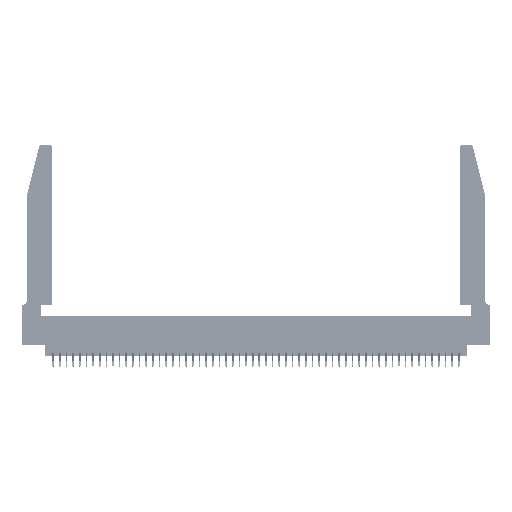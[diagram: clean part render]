
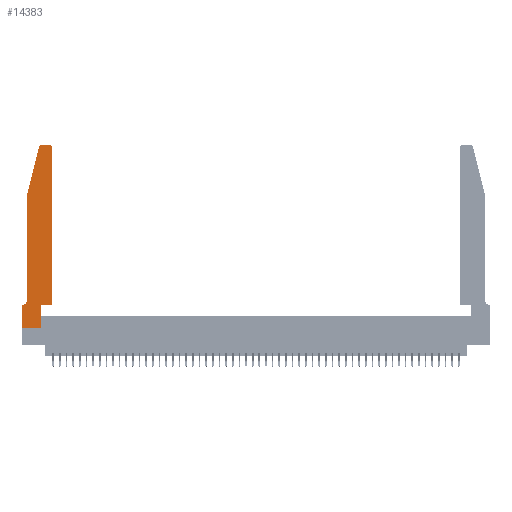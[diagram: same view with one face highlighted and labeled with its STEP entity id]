
A CAD part, top view. The second image highlights one B-rep face of the part: STEP entity #14383.
In plain terms, the highlighted planar face has unit normal (0, 0, 1).
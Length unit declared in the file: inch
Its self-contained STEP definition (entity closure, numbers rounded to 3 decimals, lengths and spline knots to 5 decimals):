
#1143 = CARTESIAN_POINT ( 'NONE',  ( 0.0755, 0.42, 0.37 ) ) ;
#2028 = DIRECTION ( 'NONE',  ( 0., 0., 1. ) ) ;
#2454 = ORIENTED_EDGE ( 'NONE', *, *, #25500, .T. ) ;
#2804 = EDGE_CURVE ( 'NONE', #31551, #34069, #6048, .T. ) ;
#2999 = EDGE_CURVE ( 'NONE', #5191, #14008, #40572, .T. ) ;
#3067 = DIRECTION ( 'NONE',  ( -0.239, -0.971, 0. ) ) ;
#3151 = CARTESIAN_POINT ( 'NONE',  ( 0.0755, 0.35, 0.37 ) ) ;
#3518 = AXIS2_PLACEMENT_3D ( 'NONE', #34191, #10553, #38124 ) ;
#3556 = VERTEX_POINT ( 'NONE', #25997 ) ;
#3999 = EDGE_LOOP ( 'NONE', ( #34614, #4310, #8051, #2454, #29791, #9944, #42616, #12453, #47513, #5003, #26138, #18088 ) ) ;
#4310 = ORIENTED_EDGE ( 'NONE', *, *, #16962, .T. ) ;
#4603 = AXIS2_PLACEMENT_3D ( 'NONE', #25837, #2028, #29796 ) ;
#5003 = ORIENTED_EDGE ( 'NONE', *, *, #2804, .T. ) ;
#5191 = VERTEX_POINT ( 'NONE', #32025 ) ;
#6048 = LINE ( 'NONE', #21754, #7297 ) ;
#6555 = PLANE ( 'NONE',  #3518 ) ;
#6983 = CARTESIAN_POINT ( 'NONE',  ( 0.2605, 2.75, 0.37 ) ) ;
#7101 = EDGE_CURVE ( 'NONE', #43563, #31551, #26178, .T. ) ;
#7297 = VECTOR ( 'NONE', #9914, 39.37008 ) ;
#7477 = LINE ( 'NONE', #26869, #37720 ) ;
#8051 = ORIENTED_EDGE ( 'NONE', *, *, #47389, .T. ) ;
#8503 = DIRECTION ( 'NONE',  ( 0., 0., -1. ) ) ;
#8507 = VERTEX_POINT ( 'NONE', #35699 ) ;
#9914 = DIRECTION ( 'NONE',  ( 1., 0., 0. ) ) ;
#9944 = ORIENTED_EDGE ( 'NONE', *, *, #44230, .T. ) ;
#10089 = EDGE_CURVE ( 'NONE', #35684, #3556, #35107, .T. ) ;
#10257 = CARTESIAN_POINT ( 'NONE',  ( 0.4205, 2.72, 0.37 ) ) ;
#10553 = DIRECTION ( 'NONE',  ( 0., 0., 1. ) ) ;
#10909 = CARTESIAN_POINT ( 'NONE',  ( 0.0755, 2., 0.37 ) ) ;
#11151 = DIRECTION ( 'NONE',  ( 0., 1., 0. ) ) ;
#12453 = ORIENTED_EDGE ( 'NONE', *, *, #48318, .T. ) ;
#12733 = LINE ( 'NONE', #19677, #32492 ) ;
#14008 = VERTEX_POINT ( 'NONE', #43639 ) ;
#14261 = DIRECTION ( 'NONE',  ( 1., 0., 0. ) ) ;
#14383 = ADVANCED_FACE ( 'NONE', ( #47519 ), #6555, .T. ) ;
#15183 = DIRECTION ( 'NONE',  ( -1., 0., 0. ) ) ;
#16836 = VERTEX_POINT ( 'NONE', #1143 ) ;
#16962 = EDGE_CURVE ( 'NONE', #3556, #35277, #45431, .T. ) ;
#18088 = ORIENTED_EDGE ( 'NONE', *, *, #19020, .T. ) ;
#18492 = VECTOR ( 'NONE', #22938, 39.37008 ) ;
#18789 = CARTESIAN_POINT ( 'NONE',  ( 0.4205, 2.75, 0.37 ) ) ;
#18971 = CARTESIAN_POINT ( 'NONE',  ( 0.25487, 2.72718, 0.37 ) ) ;
#18990 = CARTESIAN_POINT ( 'NONE',  ( 0.2865, 0.35, 0.37 ) ) ;
#19020 = EDGE_CURVE ( 'NONE', #8507, #35684, #40999, .T. ) ;
#19677 = CARTESIAN_POINT ( 'NONE',  ( 0.4505, 0.35, 0.37 ) ) ;
#21297 = EDGE_CURVE ( 'NONE', #16836, #31714, #43798, .T. ) ;
#21754 = CARTESIAN_POINT ( 'NONE',  ( 0.4505, 0.35, 0.37 ) ) ;
#22223 = DIRECTION ( 'NONE',  ( 0., -1., 0. ) ) ;
#22422 = DIRECTION ( 'NONE',  ( 1., 0., 0. ) ) ;
#22938 = DIRECTION ( 'NONE',  ( 0., -1., 0. ) ) ;
#25500 = EDGE_CURVE ( 'NONE', #47380, #16836, #27535, .T. ) ;
#25837 = CARTESIAN_POINT ( 'NONE',  ( 0.284, 2.72, 0.37 ) ) ;
#25993 = AXIS2_PLACEMENT_3D ( 'NONE', #10257, #37832, #14261 ) ;
#25997 = CARTESIAN_POINT ( 'NONE',  ( 0.284, 2.75, 0.37 ) ) ;
#26138 = ORIENTED_EDGE ( 'NONE', *, *, #37621, .T. ) ;
#26178 = LINE ( 'NONE', #18990, #36567 ) ;
#26296 = VECTOR ( 'NONE', #22223, 39.37008 ) ;
#26869 = CARTESIAN_POINT ( 'NONE',  ( 0.0755, 2., 0.37 ) ) ;
#27245 = VECTOR ( 'NONE', #22422, 39.37008 ) ;
#27535 = LINE ( 'NONE', #29981, #26296 ) ;
#29791 = ORIENTED_EDGE ( 'NONE', *, *, #21297, .T. ) ;
#29796 = DIRECTION ( 'NONE',  ( 1., 0., 0. ) ) ;
#29981 = CARTESIAN_POINT ( 'NONE',  ( 0.0755, 2., 0.37 ) ) ;
#31551 = VERTEX_POINT ( 'NONE', #49388 ) ;
#31714 = VERTEX_POINT ( 'NONE', #38798 ) ;
#32025 = CARTESIAN_POINT ( 'NONE',  ( 0., 0.35, 0.37 ) ) ;
#32199 = CARTESIAN_POINT ( 'NONE',  ( 0.0055, 0.42, 0.37 ) ) ;
#32492 = VECTOR ( 'NONE', #50989, 39.37008 ) ;
#33883 = VECTOR ( 'NONE', #38519, 39.37008 ) ;
#34069 = VERTEX_POINT ( 'NONE', #44837 ) ;
#34191 = CARTESIAN_POINT ( 'NONE',  ( 0., 0.35, 0.37 ) ) ;
#34231 = CARTESIAN_POINT ( 'NONE',  ( 0., 0., 0.37 ) ) ;
#34614 = ORIENTED_EDGE ( 'NONE', *, *, #10089, .T. ) ;
#35107 = LINE ( 'NONE', #6983, #33883 ) ;
#35277 = VERTEX_POINT ( 'NONE', #18971 ) ;
#35684 = VERTEX_POINT ( 'NONE', #18789 ) ;
#35699 = CARTESIAN_POINT ( 'NONE',  ( 0.4505, 2.72, 0.37 ) ) ;
#36109 = DIRECTION ( 'NONE',  ( -1., 0., 0. ) ) ;
#36567 = VECTOR ( 'NONE', #11151, 39.37008 ) ;
#37621 = EDGE_CURVE ( 'NONE', #34069, #8507, #12733, .T. ) ;
#37720 = VECTOR ( 'NONE', #3067, 39.37008 ) ;
#37832 = DIRECTION ( 'NONE',  ( 0., 0., 1. ) ) ;
#38124 = DIRECTION ( 'NONE',  ( 1., 0., 0. ) ) ;
#38502 = CARTESIAN_POINT ( 'NONE',  ( 0., 0., 0.37 ) ) ;
#38519 = DIRECTION ( 'NONE',  ( -1., 0., 0. ) ) ;
#38798 = CARTESIAN_POINT ( 'NONE',  ( 0.0055, 0.35, 0.37 ) ) ;
#40083 = LINE ( 'NONE', #3151, #49257 ) ;
#40572 = LINE ( 'NONE', #38502, #18492 ) ;
#40999 = CIRCLE ( 'NONE', #25993, 0.03 ) ;
#42616 = ORIENTED_EDGE ( 'NONE', *, *, #2999, .T. ) ;
#42903 = CARTESIAN_POINT ( 'NONE',  ( 0.2865, 0., 0.37 ) ) ;
#43563 = VERTEX_POINT ( 'NONE', #42903 ) ;
#43639 = CARTESIAN_POINT ( 'NONE',  ( 0., 0., 0.37 ) ) ;
#43798 = CIRCLE ( 'NONE', #48926, 0.07 ) ;
#44230 = EDGE_CURVE ( 'NONE', #31714, #5191, #40083, .T. ) ;
#44837 = CARTESIAN_POINT ( 'NONE',  ( 0.4505, 0.35, 0.37 ) ) ;
#45431 = CIRCLE ( 'NONE', #4603, 0.03 ) ;
#46796 = LINE ( 'NONE', #34231, #27245 ) ;
#47380 = VERTEX_POINT ( 'NONE', #10909 ) ;
#47389 = EDGE_CURVE ( 'NONE', #35277, #47380, #7477, .T. ) ;
#47513 = ORIENTED_EDGE ( 'NONE', *, *, #7101, .T. ) ;
#47519 = FACE_OUTER_BOUND ( 'NONE', #3999, .T. ) ;
#48318 = EDGE_CURVE ( 'NONE', #14008, #43563, #46796, .T. ) ;
#48926 = AXIS2_PLACEMENT_3D ( 'NONE', #32199, #8503, #36109 ) ;
#49257 = VECTOR ( 'NONE', #15183, 39.37008 ) ;
#49388 = CARTESIAN_POINT ( 'NONE',  ( 0.2865, 0.35, 0.37 ) ) ;
#50989 = DIRECTION ( 'NONE',  ( 0., 1., 0. ) ) ;
